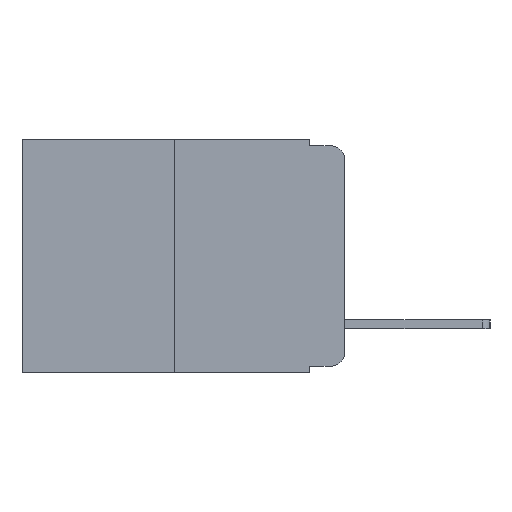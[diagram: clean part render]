
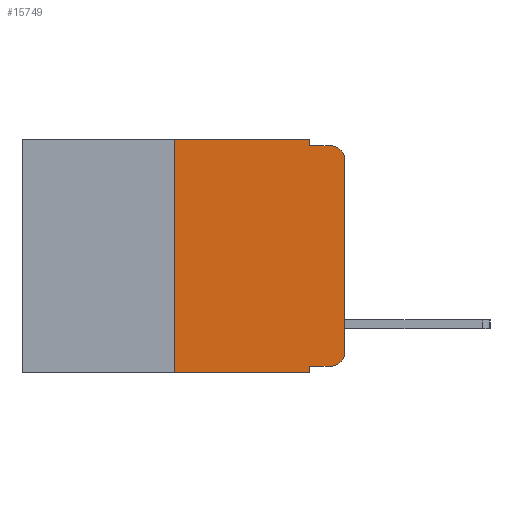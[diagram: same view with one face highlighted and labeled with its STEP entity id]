
A CAD part, left-side view. The second image highlights one B-rep face of the part: STEP entity #15749.
In plain terms, the highlighted planar face has unit normal (-1, 0, 0).
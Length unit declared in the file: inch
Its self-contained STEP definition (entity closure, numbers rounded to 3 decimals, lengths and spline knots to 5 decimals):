
#180 = DIRECTION ( 'NONE',  ( 0., 0., -1. ) ) ;
#205 = LINE ( 'NONE', #10020, #4031 ) ;
#716 = DIRECTION ( 'NONE',  ( 0., -1., 0. ) ) ;
#1175 = VERTEX_POINT ( 'NONE', #13240 ) ;
#2081 = DIRECTION ( 'NONE',  ( 1., 0., 0. ) ) ;
#2637 = ORIENTED_EDGE ( 'NONE', *, *, #6315, .T. ) ;
#2998 = CIRCLE ( 'NONE', #18944, 0.02 ) ;
#3019 = LINE ( 'NONE', #13298, #18926 ) ;
#3046 = EDGE_CURVE ( 'NONE', #1175, #15447, #7648, .T. ) ;
#3996 = LINE ( 'NONE', #9062, #15892 ) ;
#4031 = VECTOR ( 'NONE', #14650, 39.37008 ) ;
#4035 = VERTEX_POINT ( 'NONE', #7065 ) ;
#4355 = DIRECTION ( 'NONE',  ( 0., 0., 1. ) ) ;
#4946 = VERTEX_POINT ( 'NONE', #7992 ) ;
#5049 = AXIS2_PLACEMENT_3D ( 'NONE', #8273, #18870, #9825 ) ;
#5193 = EDGE_CURVE ( 'NONE', #15447, #4946, #14322, .T. ) ;
#5657 = CARTESIAN_POINT ( 'NONE',  ( 0., 0., -0.313 ) ) ;
#5693 = CARTESIAN_POINT ( 'NONE',  ( 0., 0.051, -0.343 ) ) ;
#5872 = EDGE_CURVE ( 'NONE', #11337, #13228, #3019, .T. ) ;
#5981 = CARTESIAN_POINT ( 'NONE',  ( 0., 0.051, -0.01 ) ) ;
#6315 = EDGE_CURVE ( 'NONE', #14792, #4946, #2998, .T. ) ;
#6934 = ORIENTED_EDGE ( 'NONE', *, *, #5193, .F. ) ;
#6965 = VECTOR ( 'NONE', #7919, 39.37008 ) ;
#7065 = CARTESIAN_POINT ( 'NONE',  ( 0., 0.02, -0.333 ) ) ;
#7128 = CARTESIAN_POINT ( 'NONE',  ( 0., 0.25, 0. ) ) ;
#7159 = DIRECTION ( 'NONE',  ( 0., -1., 0. ) ) ;
#7178 = CARTESIAN_POINT ( 'NONE',  ( 0., 0., -0.03 ) ) ;
#7361 = EDGE_CURVE ( 'NONE', #17956, #14792, #3996, .T. ) ;
#7648 = LINE ( 'NONE', #10209, #11300 ) ;
#7670 = FACE_OUTER_BOUND ( 'NONE', #9304, .T. ) ;
#7826 = LINE ( 'NONE', #15192, #15500 ) ;
#7919 = DIRECTION ( 'NONE',  ( 0., -1., 0. ) ) ;
#7992 = CARTESIAN_POINT ( 'NONE',  ( 0., 0.02, -0.01 ) ) ;
#8273 = CARTESIAN_POINT ( 'NONE',  ( 0., 0.02, -0.313 ) ) ;
#8422 = PLANE ( 'NONE',  #16968 ) ;
#9062 = CARTESIAN_POINT ( 'NONE',  ( 0., 0., 0. ) ) ;
#9304 = EDGE_LOOP ( 'NONE', ( #13245, #2637, #6934, #11575, #15582, #9349, #9848, #13953, #19267, #19725 ) ) ;
#9349 = ORIENTED_EDGE ( 'NONE', *, *, #19970, .F. ) ;
#9748 = DIRECTION ( 'NONE',  ( -1., 0., 0. ) ) ;
#9825 = DIRECTION ( 'NONE',  ( 0., 0., -1. ) ) ;
#9848 = ORIENTED_EDGE ( 'NONE', *, *, #5872, .T. ) ;
#9918 = VECTOR ( 'NONE', #16340, 39.37008 ) ;
#10020 = CARTESIAN_POINT ( 'NONE',  ( 0., 0.473, 0. ) ) ;
#10209 = CARTESIAN_POINT ( 'NONE',  ( 0., 0.051, 0. ) ) ;
#10680 = VERTEX_POINT ( 'NONE', #13468 ) ;
#10992 = CARTESIAN_POINT ( 'NONE',  ( 0., 0.25, 0. ) ) ;
#11123 = LINE ( 'NONE', #18535, #6965 ) ;
#11300 = VECTOR ( 'NONE', #13667, 39.37008 ) ;
#11337 = VERTEX_POINT ( 'NONE', #18269 ) ;
#11575 = ORIENTED_EDGE ( 'NONE', *, *, #3046, .F. ) ;
#11577 = CARTESIAN_POINT ( 'NONE',  ( 0., 0.473, 0. ) ) ;
#12352 = EDGE_CURVE ( 'NONE', #4035, #17956, #13524, .T. ) ;
#12864 = EDGE_CURVE ( 'NONE', #10680, #4035, #11123, .T. ) ;
#13117 = DIRECTION ( 'NONE',  ( 0., 0., -1. ) ) ;
#13228 = VERTEX_POINT ( 'NONE', #5693 ) ;
#13240 = CARTESIAN_POINT ( 'NONE',  ( 0., 0.051, 0. ) ) ;
#13245 = ORIENTED_EDGE ( 'NONE', *, *, #7361, .T. ) ;
#13298 = CARTESIAN_POINT ( 'NONE',  ( 0., 0.473, -0.343 ) ) ;
#13468 = CARTESIAN_POINT ( 'NONE',  ( 0., 0.051, -0.333 ) ) ;
#13524 = CIRCLE ( 'NONE', #5049, 0.02 ) ;
#13667 = DIRECTION ( 'NONE',  ( 0., 0., -1. ) ) ;
#13953 = ORIENTED_EDGE ( 'NONE', *, *, #17559, .F. ) ;
#14322 = LINE ( 'NONE', #17807, #18267 ) ;
#14490 = LINE ( 'NONE', #7128, #9918 ) ;
#14650 = DIRECTION ( 'NONE',  ( 0., -1., 0. ) ) ;
#14694 = EDGE_CURVE ( 'NONE', #19013, #1175, #205, .T. ) ;
#14792 = VERTEX_POINT ( 'NONE', #7178 ) ;
#15192 = CARTESIAN_POINT ( 'NONE',  ( 0., 0.051, 0. ) ) ;
#15447 = VERTEX_POINT ( 'NONE', #5981 ) ;
#15500 = VECTOR ( 'NONE', #16683, 39.37008 ) ;
#15582 = ORIENTED_EDGE ( 'NONE', *, *, #14694, .F. ) ;
#15749 = ADVANCED_FACE ( 'NONE', ( #7670 ), #8422, .F. ) ;
#15892 = VECTOR ( 'NONE', #4355, 39.37008 ) ;
#16340 = DIRECTION ( 'NONE',  ( 0., 0., 1. ) ) ;
#16683 = DIRECTION ( 'NONE',  ( 0., 0., -1. ) ) ;
#16968 = AXIS2_PLACEMENT_3D ( 'NONE', #11577, #2081, #13117 ) ;
#17559 = EDGE_CURVE ( 'NONE', #10680, #13228, #7826, .T. ) ;
#17807 = CARTESIAN_POINT ( 'NONE',  ( 0., 0.051, -0.01 ) ) ;
#17956 = VERTEX_POINT ( 'NONE', #5657 ) ;
#18267 = VECTOR ( 'NONE', #7159, 39.37008 ) ;
#18269 = CARTESIAN_POINT ( 'NONE',  ( 0., 0.25, -0.343 ) ) ;
#18535 = CARTESIAN_POINT ( 'NONE',  ( 0., 0.051, -0.333 ) ) ;
#18806 = CARTESIAN_POINT ( 'NONE',  ( 0., 0.02, -0.03 ) ) ;
#18870 = DIRECTION ( 'NONE',  ( -1., 0., 0. ) ) ;
#18926 = VECTOR ( 'NONE', #716, 39.37008 ) ;
#18944 = AXIS2_PLACEMENT_3D ( 'NONE', #18806, #9748, #180 ) ;
#19013 = VERTEX_POINT ( 'NONE', #10992 ) ;
#19267 = ORIENTED_EDGE ( 'NONE', *, *, #12864, .T. ) ;
#19725 = ORIENTED_EDGE ( 'NONE', *, *, #12352, .T. ) ;
#19970 = EDGE_CURVE ( 'NONE', #11337, #19013, #14490, .T. ) ;
